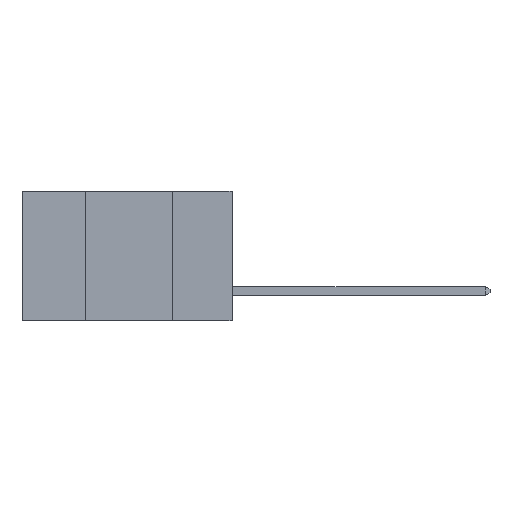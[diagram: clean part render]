
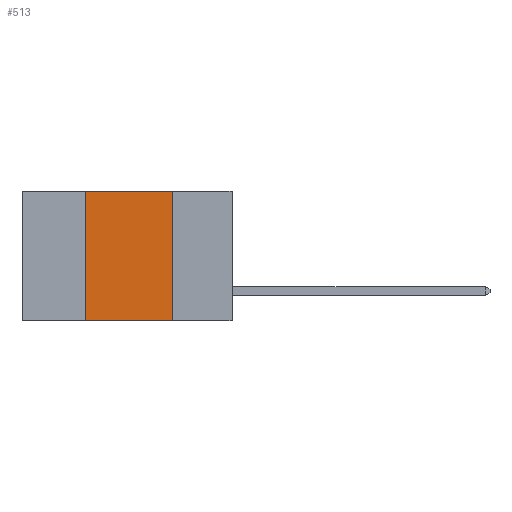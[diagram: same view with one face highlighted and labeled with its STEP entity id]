
A CAD part, left-side view. The second image highlights one B-rep face of the part: STEP entity #513.
In plain terms, the highlighted planar face has unit normal (-1, 0, 0).
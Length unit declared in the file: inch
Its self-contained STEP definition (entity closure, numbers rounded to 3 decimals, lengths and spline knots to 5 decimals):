
#279 = EDGE_CURVE ( 'NONE', #6716, #12558, #558, .T. ) ;
#513 = ADVANCED_FACE ( 'NONE', ( #7792 ), #15758, .F. ) ;
#558 = LINE ( 'NONE', #7750, #10695 ) ;
#1621 = CARTESIAN_POINT ( 'NONE',  ( 0., 0.6, 0. ) ) ;
#2153 = DIRECTION ( 'NONE',  ( 1., 0., 0. ) ) ;
#2154 = EDGE_CURVE ( 'NONE', #12558, #9214, #3494, .T. ) ;
#3351 = DIRECTION ( 'NONE',  ( 0., 0., -1. ) ) ;
#3494 = LINE ( 'NONE', #12846, #6529 ) ;
#3846 = AXIS2_PLACEMENT_3D ( 'NONE', #1621, #2153, #3351 ) ;
#3907 = DIRECTION ( 'NONE',  ( 0., 0., 1. ) ) ;
#4637 = CARTESIAN_POINT ( 'NONE',  ( 0., 0.17, -0.37 ) ) ;
#5550 = DIRECTION ( 'NONE',  ( 0., -1., 0. ) ) ;
#6191 = VECTOR ( 'NONE', #3907, 39.37008 ) ;
#6363 = CARTESIAN_POINT ( 'NONE',  ( 0., 0.6, -0.37 ) ) ;
#6510 = CARTESIAN_POINT ( 'NONE',  ( 0., 0.42, 0. ) ) ;
#6529 = VECTOR ( 'NONE', #12939, 39.37008 ) ;
#6601 = LINE ( 'NONE', #6510, #6191 ) ;
#6716 = VERTEX_POINT ( 'NONE', #8410 ) ;
#7622 = VECTOR ( 'NONE', #14846, 39.37008 ) ;
#7750 = CARTESIAN_POINT ( 'NONE',  ( 0., 0.6, 0. ) ) ;
#7792 = FACE_OUTER_BOUND ( 'NONE', #12914, .T. ) ;
#7865 = ORIENTED_EDGE ( 'NONE', *, *, #10264, .F. ) ;
#8393 = ORIENTED_EDGE ( 'NONE', *, *, #9466, .T. ) ;
#8410 = CARTESIAN_POINT ( 'NONE',  ( 0., 0.42, 0. ) ) ;
#9214 = VERTEX_POINT ( 'NONE', #4637 ) ;
#9466 = EDGE_CURVE ( 'NONE', #12187, #9214, #10881, .T. ) ;
#10264 = EDGE_CURVE ( 'NONE', #12187, #6716, #6601, .T. ) ;
#10695 = VECTOR ( 'NONE', #5550, 39.37008 ) ;
#10881 = LINE ( 'NONE', #6363, #7622 ) ;
#11622 = ORIENTED_EDGE ( 'NONE', *, *, #2154, .F. ) ;
#12187 = VERTEX_POINT ( 'NONE', #15127 ) ;
#12558 = VERTEX_POINT ( 'NONE', #13112 ) ;
#12846 = CARTESIAN_POINT ( 'NONE',  ( 0., 0.17, 0. ) ) ;
#12914 = EDGE_LOOP ( 'NONE', ( #11622, #15870, #7865, #8393 ) ) ;
#12939 = DIRECTION ( 'NONE',  ( 0., 0., -1. ) ) ;
#13112 = CARTESIAN_POINT ( 'NONE',  ( 0., 0.17, 0. ) ) ;
#14846 = DIRECTION ( 'NONE',  ( 0., -1., 0. ) ) ;
#15127 = CARTESIAN_POINT ( 'NONE',  ( 0., 0.42, -0.37 ) ) ;
#15758 = PLANE ( 'NONE',  #3846 ) ;
#15870 = ORIENTED_EDGE ( 'NONE', *, *, #279, .F. ) ;
